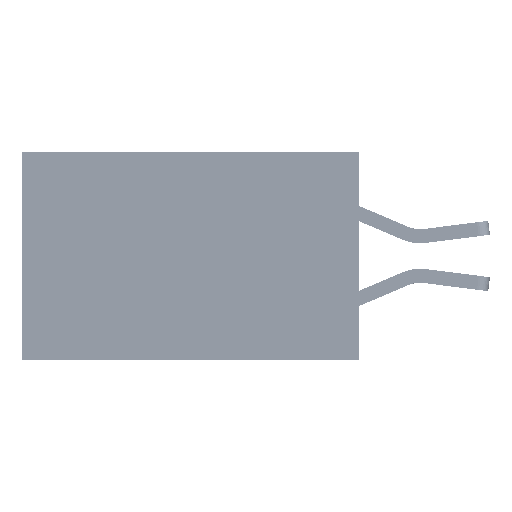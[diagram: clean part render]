
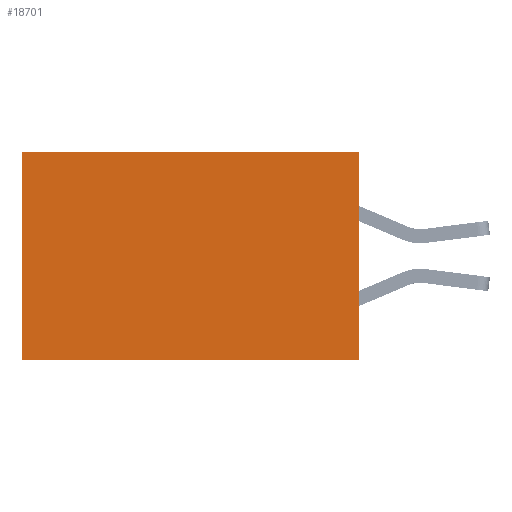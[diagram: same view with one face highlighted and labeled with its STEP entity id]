
A CAD part, left-side view. The second image highlights one B-rep face of the part: STEP entity #18701.
In plain terms, the highlighted planar face has unit normal (-1, 0, 0).
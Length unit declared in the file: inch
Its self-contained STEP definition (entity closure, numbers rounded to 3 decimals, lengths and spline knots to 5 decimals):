
#868 = CARTESIAN_POINT ( 'NONE',  ( 0.2875, 0., 0. ) ) ;
#899 = EDGE_LOOP ( 'NONE', ( #2482, #34214, #1743, #31689 ) ) ;
#1657 = VECTOR ( 'NONE', #23608, 39.37008 ) ;
#1743 = ORIENTED_EDGE ( 'NONE', *, *, #37420, .F. ) ;
#2234 = DIRECTION ( 'NONE',  ( 0., 0., -1. ) ) ;
#2482 = ORIENTED_EDGE ( 'NONE', *, *, #20975, .T. ) ;
#3968 = VECTOR ( 'NONE', #9772, 39.37008 ) ;
#6110 = CARTESIAN_POINT ( 'NONE',  ( 0.2875, 0., -0.37 ) ) ;
#9666 = CARTESIAN_POINT ( 'NONE',  ( 0.2875, 0., 0. ) ) ;
#9772 = DIRECTION ( 'NONE',  ( 0., 0., -1. ) ) ;
#11487 = CARTESIAN_POINT ( 'NONE',  ( 0.2875, 0.6, 0. ) ) ;
#11803 = DIRECTION ( 'NONE',  ( 1., 0., 0. ) ) ;
#12568 = FACE_OUTER_BOUND ( 'NONE', #899, .T. ) ;
#13198 = CARTESIAN_POINT ( 'NONE',  ( 0.2875, 0.6, 0. ) ) ;
#13332 = LINE ( 'NONE', #26664, #31711 ) ;
#18672 = VERTEX_POINT ( 'NONE', #11487 ) ;
#18701 = ADVANCED_FACE ( 'NONE', ( #12568 ), #39424, .F. ) ;
#20975 = EDGE_CURVE ( 'NONE', #18672, #38314, #23807, .T. ) ;
#23608 = DIRECTION ( 'NONE',  ( 0., 1., 0. ) ) ;
#23674 = VECTOR ( 'NONE', #26978, 39.37008 ) ;
#23698 = LINE ( 'NONE', #9666, #1657 ) ;
#23807 = LINE ( 'NONE', #13198, #3968 ) ;
#25631 = CARTESIAN_POINT ( 'NONE',  ( 0.2875, 0., -0.37 ) ) ;
#26061 = VERTEX_POINT ( 'NONE', #25631 ) ;
#26664 = CARTESIAN_POINT ( 'NONE',  ( 0.2875, 0., 0. ) ) ;
#26978 = DIRECTION ( 'NONE',  ( 0., 1., 0. ) ) ;
#29295 = VERTEX_POINT ( 'NONE', #39017 ) ;
#31689 = ORIENTED_EDGE ( 'NONE', *, *, #37496, .T. ) ;
#31711 = VECTOR ( 'NONE', #2234, 39.37008 ) ;
#32119 = EDGE_CURVE ( 'NONE', #26061, #38314, #41016, .T. ) ;
#34214 = ORIENTED_EDGE ( 'NONE', *, *, #32119, .F. ) ;
#36041 = DIRECTION ( 'NONE',  ( 0., 0., -1. ) ) ;
#37420 = EDGE_CURVE ( 'NONE', #29295, #26061, #13332, .T. ) ;
#37496 = EDGE_CURVE ( 'NONE', #29295, #18672, #23698, .T. ) ;
#38314 = VERTEX_POINT ( 'NONE', #40141 ) ;
#39017 = CARTESIAN_POINT ( 'NONE',  ( 0.2875, 0., 0. ) ) ;
#39424 = PLANE ( 'NONE',  #42003 ) ;
#40141 = CARTESIAN_POINT ( 'NONE',  ( 0.2875, 0.6, -0.37 ) ) ;
#41016 = LINE ( 'NONE', #6110, #23674 ) ;
#42003 = AXIS2_PLACEMENT_3D ( 'NONE', #868, #11803, #36041 ) ;
